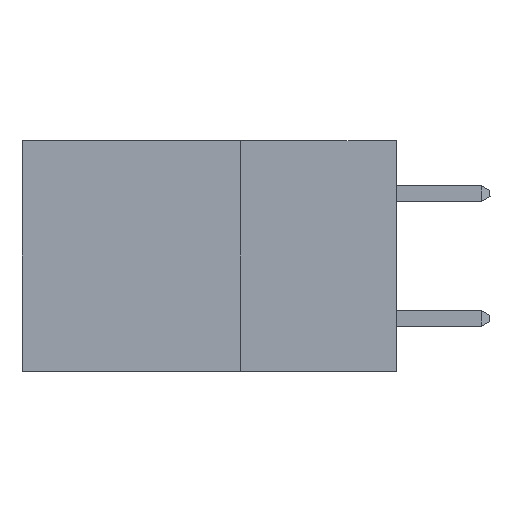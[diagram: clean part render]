
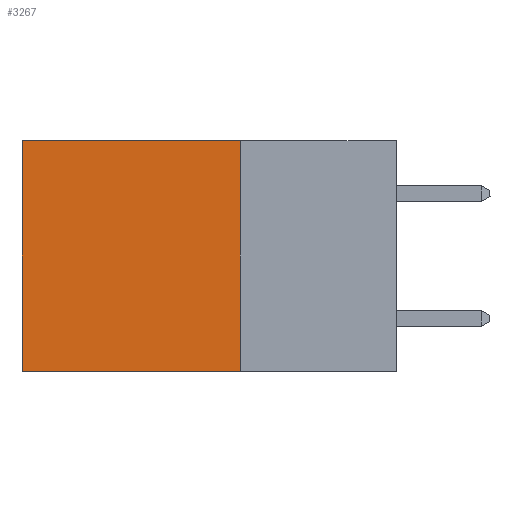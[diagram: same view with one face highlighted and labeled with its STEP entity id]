
A CAD part, left-side view. The second image highlights one B-rep face of the part: STEP entity #3267.
In plain terms, the highlighted planar face has unit normal (-1, 0, 0).
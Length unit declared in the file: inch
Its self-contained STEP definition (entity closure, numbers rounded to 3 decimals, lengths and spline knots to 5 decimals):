
#739 = EDGE_CURVE ( 'NONE', #1820, #10296, #7067, .T. ) ;
#1005 = AXIS2_PLACEMENT_3D ( 'NONE', #19614, #8717, #6769 ) ;
#1820 = VERTEX_POINT ( 'NONE', #6520 ) ;
#2242 = DIRECTION ( 'NONE',  ( 0., 1., 0. ) ) ;
#2553 = VECTOR ( 'NONE', #2672, 39.37008 ) ;
#2672 = DIRECTION ( 'NONE',  ( 0., 1., 0. ) ) ;
#3267 = ADVANCED_FACE ( 'NONE', ( #25621 ), #8802, .F. ) ;
#3781 = DIRECTION ( 'NONE',  ( 0., 0., -1. ) ) ;
#6174 = CARTESIAN_POINT ( 'NONE',  ( 0.298, 0.6, 0. ) ) ;
#6520 = CARTESIAN_POINT ( 'NONE',  ( 0.298, 0.25, 0. ) ) ;
#6769 = DIRECTION ( 'NONE',  ( 0., 0., -1. ) ) ;
#7067 = LINE ( 'NONE', #12787, #17644 ) ;
#7136 = CARTESIAN_POINT ( 'NONE',  ( 0.298, 0.25, -0.37 ) ) ;
#8717 = DIRECTION ( 'NONE',  ( 1., 0., 0. ) ) ;
#8802 = PLANE ( 'NONE',  #1005 ) ;
#10008 = ORIENTED_EDGE ( 'NONE', *, *, #739, .T. ) ;
#10082 = VECTOR ( 'NONE', #10769, 39.37008 ) ;
#10296 = VERTEX_POINT ( 'NONE', #22630 ) ;
#10652 = VERTEX_POINT ( 'NONE', #24970 ) ;
#10769 = DIRECTION ( 'NONE',  ( 0., 0., -1. ) ) ;
#11552 = LINE ( 'NONE', #25736, #2553 ) ;
#12787 = CARTESIAN_POINT ( 'NONE',  ( 0.298, 0.25, 0. ) ) ;
#13142 = ORIENTED_EDGE ( 'NONE', *, *, #24399, .F. ) ;
#13431 = VECTOR ( 'NONE', #3781, 39.37008 ) ;
#16242 = EDGE_CURVE ( 'NONE', #24141, #10652, #11552, .T. ) ;
#17172 = ORIENTED_EDGE ( 'NONE', *, *, #16242, .F. ) ;
#17644 = VECTOR ( 'NONE', #2242, 39.37008 ) ;
#18927 = CARTESIAN_POINT ( 'NONE',  ( 0.298, 0.25, 0. ) ) ;
#19043 = LINE ( 'NONE', #6174, #13431 ) ;
#19614 = CARTESIAN_POINT ( 'NONE',  ( 0.298, 0.25, 0. ) ) ;
#20068 = EDGE_LOOP ( 'NONE', ( #26445, #17172, #13142, #10008 ) ) ;
#22630 = CARTESIAN_POINT ( 'NONE',  ( 0.298, 0.6, 0. ) ) ;
#24141 = VERTEX_POINT ( 'NONE', #7136 ) ;
#24291 = EDGE_CURVE ( 'NONE', #10296, #10652, #19043, .T. ) ;
#24399 = EDGE_CURVE ( 'NONE', #1820, #24141, #26008, .T. ) ;
#24970 = CARTESIAN_POINT ( 'NONE',  ( 0.298, 0.6, -0.37 ) ) ;
#25621 = FACE_OUTER_BOUND ( 'NONE', #20068, .T. ) ;
#25736 = CARTESIAN_POINT ( 'NONE',  ( 0.298, 0.25, -0.37 ) ) ;
#26008 = LINE ( 'NONE', #18927, #10082 ) ;
#26445 = ORIENTED_EDGE ( 'NONE', *, *, #24291, .T. ) ;
